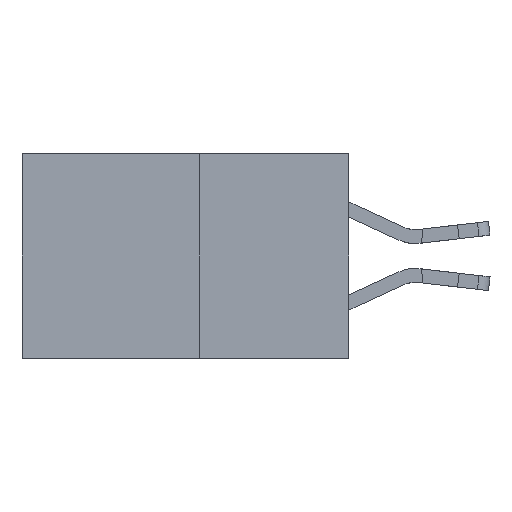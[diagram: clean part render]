
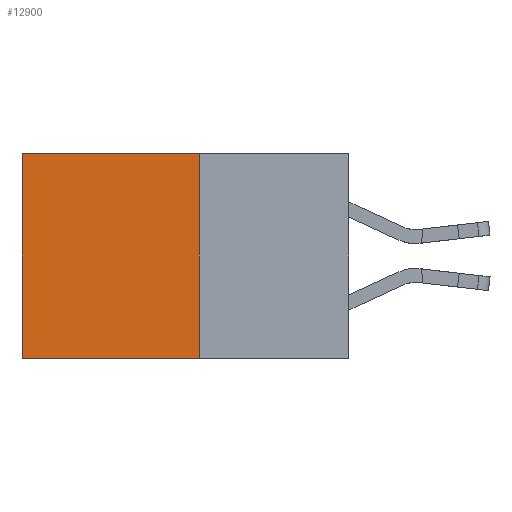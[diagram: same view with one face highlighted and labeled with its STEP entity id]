
A CAD part, left-side view. The second image highlights one B-rep face of the part: STEP entity #12900.
In plain terms, the highlighted planar face has unit normal (-1, 0, 0).
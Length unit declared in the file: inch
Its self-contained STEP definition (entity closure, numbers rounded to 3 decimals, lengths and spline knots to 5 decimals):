
#93 = LINE ( 'NONE', #15415, #17071 ) ;
#363 = PLANE ( 'NONE',  #17242 ) ;
#977 = CARTESIAN_POINT ( 'NONE',  ( 0.277, 0.27, 0. ) ) ;
#2048 = CARTESIAN_POINT ( 'NONE',  ( 0.277, 0.27, -0.37 ) ) ;
#2936 = VECTOR ( 'NONE', #17331, 39.37008 ) ;
#3141 = VERTEX_POINT ( 'NONE', #19434 ) ;
#3350 = FACE_OUTER_BOUND ( 'NONE', #6037, .T. ) ;
#4002 = ORIENTED_EDGE ( 'NONE', *, *, #19010, .F. ) ;
#4442 = CARTESIAN_POINT ( 'NONE',  ( 0.277, 0.59, 0. ) ) ;
#5241 = CARTESIAN_POINT ( 'NONE',  ( 0.277, 0.27, 0. ) ) ;
#5398 = VECTOR ( 'NONE', #20940, 39.37008 ) ;
#5505 = ORIENTED_EDGE ( 'NONE', *, *, #16917, .T. ) ;
#5745 = LINE ( 'NONE', #10353, #13969 ) ;
#6037 = EDGE_LOOP ( 'NONE', ( #10572, #4002, #18902, #5505 ) ) ;
#6972 = DIRECTION ( 'NONE',  ( 0., 0., -1. ) ) ;
#9665 = EDGE_CURVE ( 'NONE', #9882, #3141, #93, .T. ) ;
#9882 = VERTEX_POINT ( 'NONE', #4442 ) ;
#10271 = EDGE_CURVE ( 'NONE', #19966, #10619, #5745, .T. ) ;
#10353 = CARTESIAN_POINT ( 'NONE',  ( 0.277, 0.27, -0.37 ) ) ;
#10535 = DIRECTION ( 'NONE',  ( 0., 0., -1. ) ) ;
#10572 = ORIENTED_EDGE ( 'NONE', *, *, #9665, .T. ) ;
#10619 = VERTEX_POINT ( 'NONE', #16096 ) ;
#12900 = ADVANCED_FACE ( 'NONE', ( #3350 ), #363, .F. ) ;
#13969 = VECTOR ( 'NONE', #18543, 39.37008 ) ;
#14125 = LINE ( 'NONE', #19310, #5398 ) ;
#15415 = CARTESIAN_POINT ( 'NONE',  ( 0.277, 0.59, -0.37 ) ) ;
#16096 = CARTESIAN_POINT ( 'NONE',  ( 0.277, 0.27, -0.37 ) ) ;
#16820 = DIRECTION ( 'NONE',  ( 1., 0., 0. ) ) ;
#16917 = EDGE_CURVE ( 'NONE', #19966, #9882, #19839, .T. ) ;
#17071 = VECTOR ( 'NONE', #10535, 39.37008 ) ;
#17242 = AXIS2_PLACEMENT_3D ( 'NONE', #2048, #16820, #6972 ) ;
#17331 = DIRECTION ( 'NONE',  ( 0., 1., 0. ) ) ;
#18543 = DIRECTION ( 'NONE',  ( 0., 0., -1. ) ) ;
#18902 = ORIENTED_EDGE ( 'NONE', *, *, #10271, .F. ) ;
#19010 = EDGE_CURVE ( 'NONE', #10619, #3141, #14125, .T. ) ;
#19310 = CARTESIAN_POINT ( 'NONE',  ( 0.277, 0.27, -0.37 ) ) ;
#19434 = CARTESIAN_POINT ( 'NONE',  ( 0.277, 0.59, -0.37 ) ) ;
#19839 = LINE ( 'NONE', #977, #2936 ) ;
#19966 = VERTEX_POINT ( 'NONE', #5241 ) ;
#20940 = DIRECTION ( 'NONE',  ( 0., 1., 0. ) ) ;
